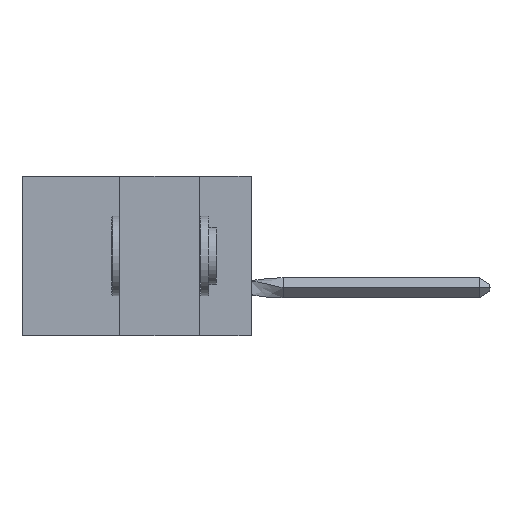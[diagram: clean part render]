
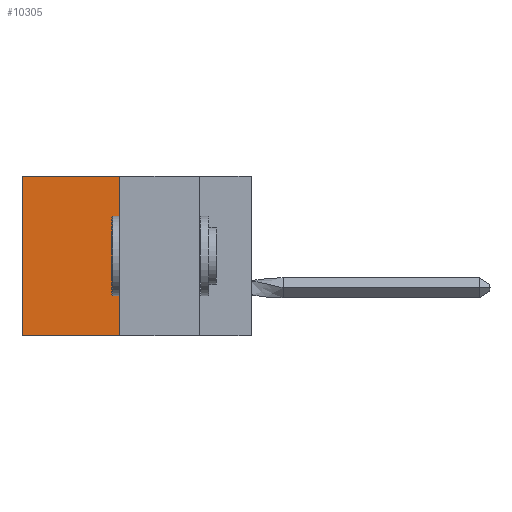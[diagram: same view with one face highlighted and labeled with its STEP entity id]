
A CAD part, left-side view. The second image highlights one B-rep face of the part: STEP entity #10305.
In plain terms, the highlighted planar face has unit normal (-1, 0, 0).
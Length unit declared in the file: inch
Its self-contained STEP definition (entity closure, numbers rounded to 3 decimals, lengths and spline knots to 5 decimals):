
#77 = CARTESIAN_POINT ( 'NONE',  ( 0.305, 0.72, 0. ) ) ;
#113 = CARTESIAN_POINT ( 'NONE',  ( 0.305, 0.413, -0.5 ) ) ;
#204 = CARTESIAN_POINT ( 'NONE',  ( 0.305, 0.413, 0. ) ) ;
#481 = EDGE_LOOP ( 'NONE', ( #7372, #7754, #8730, #8937 ) ) ;
#946 = VECTOR ( 'NONE', #3329, 39.37008 ) ;
#1680 = DIRECTION ( 'NONE',  ( 0., 1., 0. ) ) ;
#1709 = VERTEX_POINT ( 'NONE', #204 ) ;
#1803 = CARTESIAN_POINT ( 'NONE',  ( 0.305, 0.413, 0. ) ) ;
#1948 = CARTESIAN_POINT ( 'NONE',  ( 0.305, 0.72, -0.5 ) ) ;
#2180 = DIRECTION ( 'NONE',  ( 0., 0., -1. ) ) ;
#2602 = VERTEX_POINT ( 'NONE', #7849 ) ;
#2879 = PLANE ( 'NONE',  #4051 ) ;
#3083 = DIRECTION ( 'NONE',  ( 0., 0., -1. ) ) ;
#3181 = CARTESIAN_POINT ( 'NONE',  ( 0.305, 0.413, -0.5 ) ) ;
#3329 = DIRECTION ( 'NONE',  ( 0., 1., 0. ) ) ;
#3756 = FACE_OUTER_BOUND ( 'NONE', #481, .T. ) ;
#3815 = LINE ( 'NONE', #4452, #946 ) ;
#3983 = VERTEX_POINT ( 'NONE', #4349 ) ;
#4051 = AXIS2_PLACEMENT_3D ( 'NONE', #113, #4191, #2180 ) ;
#4191 = DIRECTION ( 'NONE',  ( 1., 0., 0. ) ) ;
#4349 = CARTESIAN_POINT ( 'NONE',  ( 0.305, 0.413, -0.5 ) ) ;
#4452 = CARTESIAN_POINT ( 'NONE',  ( 0.305, 0.413, -0.5 ) ) ;
#6986 = DIRECTION ( 'NONE',  ( 0., 0., -1. ) ) ;
#7002 = EDGE_CURVE ( 'NONE', #1709, #3983, #10551, .T. ) ;
#7372 = ORIENTED_EDGE ( 'NONE', *, *, #7466, .T. ) ;
#7466 = EDGE_CURVE ( 'NONE', #11488, #2602, #8936, .T. ) ;
#7652 = LINE ( 'NONE', #1803, #8129 ) ;
#7754 = ORIENTED_EDGE ( 'NONE', *, *, #8275, .F. ) ;
#7849 = CARTESIAN_POINT ( 'NONE',  ( 0.305, 0.72, -0.5 ) ) ;
#7938 = EDGE_CURVE ( 'NONE', #1709, #11488, #7652, .T. ) ;
#7982 = VECTOR ( 'NONE', #6986, 39.37008 ) ;
#8129 = VECTOR ( 'NONE', #1680, 39.37008 ) ;
#8275 = EDGE_CURVE ( 'NONE', #3983, #2602, #3815, .T. ) ;
#8730 = ORIENTED_EDGE ( 'NONE', *, *, #7002, .F. ) ;
#8936 = LINE ( 'NONE', #1948, #7982 ) ;
#8937 = ORIENTED_EDGE ( 'NONE', *, *, #7938, .T. ) ;
#10305 = ADVANCED_FACE ( 'NONE', ( #3756 ), #2879, .F. ) ;
#10551 = LINE ( 'NONE', #3181, #12283 ) ;
#11488 = VERTEX_POINT ( 'NONE', #77 ) ;
#12283 = VECTOR ( 'NONE', #3083, 39.37008 ) ;
